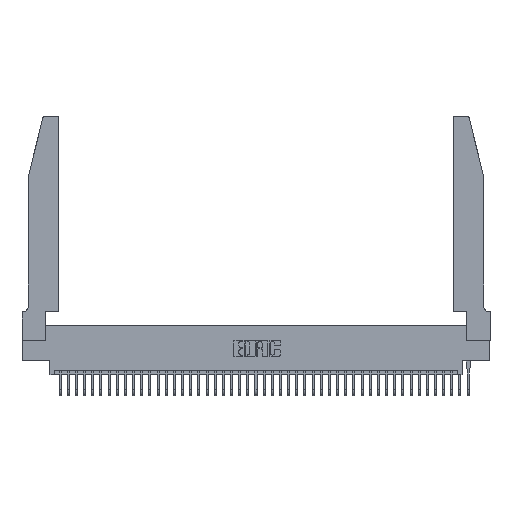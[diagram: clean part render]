
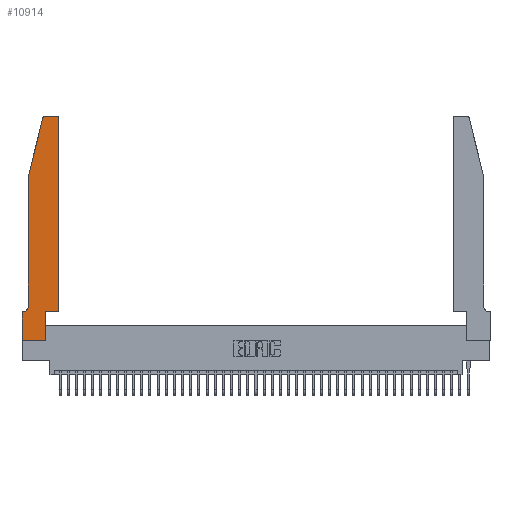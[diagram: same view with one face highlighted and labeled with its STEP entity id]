
A CAD part, top view. The second image highlights one B-rep face of the part: STEP entity #10914.
In plain terms, the highlighted planar face has unit normal (0, 0, 1).
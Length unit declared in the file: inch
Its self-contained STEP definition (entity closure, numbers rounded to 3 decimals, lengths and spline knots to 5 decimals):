
#452 = CARTESIAN_POINT ( 'NONE',  ( 0.0055, 0.35, 0.37 ) ) ;
#762 = EDGE_CURVE ( 'NONE', #5723, #13962, #36899, .T. ) ;
#776 = VERTEX_POINT ( 'NONE', #13655 ) ;
#2385 = DIRECTION ( 'NONE',  ( 1., 0., 0. ) ) ;
#2672 = CIRCLE ( 'NONE', #35893, 0.03 ) ;
#3003 = ORIENTED_EDGE ( 'NONE', *, *, #762, .T. ) ;
#4934 = EDGE_CURVE ( 'NONE', #37605, #13787, #37112, .T. ) ;
#5388 = ORIENTED_EDGE ( 'NONE', *, *, #30100, .T. ) ;
#5570 = VECTOR ( 'NONE', #32090, 39.37008 ) ;
#5597 = EDGE_CURVE ( 'NONE', #13962, #30476, #32188, .T. ) ;
#5723 = VERTEX_POINT ( 'NONE', #16733 ) ;
#6811 = ORIENTED_EDGE ( 'NONE', *, *, #8704, .T. ) ;
#6964 = VECTOR ( 'NONE', #10161, 39.37008 ) ;
#7181 = AXIS2_PLACEMENT_3D ( 'NONE', #8800, #21561, #2385 ) ;
#7262 = ORIENTED_EDGE ( 'NONE', *, *, #23439, .T. ) ;
#7342 = VECTOR ( 'NONE', #17781, 39.37008 ) ;
#8704 = EDGE_CURVE ( 'NONE', #13787, #10696, #13478, .T. ) ;
#8800 = CARTESIAN_POINT ( 'NONE',  ( 0., 0.35, 0.37 ) ) ;
#9521 = CARTESIAN_POINT ( 'NONE',  ( 0.284, 2.72, 0.37 ) ) ;
#9686 = VECTOR ( 'NONE', #13775, 39.37008 ) ;
#10075 = CARTESIAN_POINT ( 'NONE',  ( 0.284, 2.75, 0.37 ) ) ;
#10147 = CARTESIAN_POINT ( 'NONE',  ( 0.4505, 0.35, 0.37 ) ) ;
#10161 = DIRECTION ( 'NONE',  ( -1., 0., 0. ) ) ;
#10356 = VECTOR ( 'NONE', #30789, 39.37008 ) ;
#10497 = ORIENTED_EDGE ( 'NONE', *, *, #40943, .T. ) ;
#10669 = LINE ( 'NONE', #13637, #9686 ) ;
#10696 = VERTEX_POINT ( 'NONE', #14131 ) ;
#10909 = EDGE_CURVE ( 'NONE', #776, #25133, #19751, .T. ) ;
#10914 = ADVANCED_FACE ( 'NONE', ( #36312 ), #12021, .T. ) ;
#11039 = ORIENTED_EDGE ( 'NONE', *, *, #29317, .T. ) ;
#11155 = VERTEX_POINT ( 'NONE', #25811 ) ;
#11218 = ORIENTED_EDGE ( 'NONE', *, *, #27161, .T. ) ;
#11342 = LINE ( 'NONE', #40003, #10356 ) ;
#11932 = VERTEX_POINT ( 'NONE', #19848 ) ;
#12021 = PLANE ( 'NONE',  #7181 ) ;
#12068 = DIRECTION ( 'NONE',  ( 0., 0., 1. ) ) ;
#12710 = DIRECTION ( 'NONE',  ( 1., 0., 0. ) ) ;
#12932 = VECTOR ( 'NONE', #19146, 39.37008 ) ;
#13346 = CARTESIAN_POINT ( 'NONE',  ( 0.0755, 0.35, 0.37 ) ) ;
#13478 = LINE ( 'NONE', #14760, #29183 ) ;
#13637 = CARTESIAN_POINT ( 'NONE',  ( 0.2865, 0.35, 0.37 ) ) ;
#13655 = CARTESIAN_POINT ( 'NONE',  ( 0.0755, 0.42, 0.37 ) ) ;
#13775 = DIRECTION ( 'NONE',  ( 0., 1., 0. ) ) ;
#13787 = VERTEX_POINT ( 'NONE', #37447 ) ;
#13962 = VERTEX_POINT ( 'NONE', #16564 ) ;
#14131 = CARTESIAN_POINT ( 'NONE',  ( 0.4505, 2.72, 0.37 ) ) ;
#14760 = CARTESIAN_POINT ( 'NONE',  ( 0.4505, 0.35, 0.37 ) ) ;
#15422 = DIRECTION ( 'NONE',  ( -1., 0., 0. ) ) ;
#16564 = CARTESIAN_POINT ( 'NONE',  ( 0., 0., 0.37 ) ) ;
#16733 = CARTESIAN_POINT ( 'NONE',  ( 0., 0.35, 0.37 ) ) ;
#17781 = DIRECTION ( 'NONE',  ( -0.239, -0.971, 0. ) ) ;
#18431 = DIRECTION ( 'NONE',  ( 0., 0., -1. ) ) ;
#18653 = EDGE_CURVE ( 'NONE', #26326, #11155, #26989, .T. ) ;
#19146 = DIRECTION ( 'NONE',  ( 0., -1., 0. ) ) ;
#19384 = DIRECTION ( 'NONE',  ( 1., 0., 0. ) ) ;
#19490 = VECTOR ( 'NONE', #15422, 39.37008 ) ;
#19751 = CIRCLE ( 'NONE', #39539, 0.07 ) ;
#19848 = CARTESIAN_POINT ( 'NONE',  ( 0.0755, 2., 0.37 ) ) ;
#21561 = DIRECTION ( 'NONE',  ( 0., 0., 1. ) ) ;
#22442 = LINE ( 'NONE', #27901, #19490 ) ;
#22860 = ORIENTED_EDGE ( 'NONE', *, *, #5597, .T. ) ;
#23018 = EDGE_LOOP ( 'NONE', ( #10497, #25179, #11039, #7262, #34843, #11218, #3003, #22860, #30394, #24170, #6811, #5388 ) ) ;
#23439 = EDGE_CURVE ( 'NONE', #11932, #776, #11342, .T. ) ;
#23904 = CARTESIAN_POINT ( 'NONE',  ( 0.4205, 2.75, 0.37 ) ) ;
#23949 = CARTESIAN_POINT ( 'NONE',  ( 0.0755, 2., 0.37 ) ) ;
#24170 = ORIENTED_EDGE ( 'NONE', *, *, #4934, .T. ) ;
#24412 = AXIS2_PLACEMENT_3D ( 'NONE', #9521, #31472, #12710 ) ;
#25133 = VERTEX_POINT ( 'NONE', #452 ) ;
#25179 = ORIENTED_EDGE ( 'NONE', *, *, #18653, .T. ) ;
#25811 = CARTESIAN_POINT ( 'NONE',  ( 0.25487, 2.72718, 0.37 ) ) ;
#26326 = VERTEX_POINT ( 'NONE', #10075 ) ;
#26375 = CARTESIAN_POINT ( 'NONE',  ( 0.2865, 0., 0.37 ) ) ;
#26989 = CIRCLE ( 'NONE', #24412, 0.03 ) ;
#27161 = EDGE_CURVE ( 'NONE', #25133, #5723, #32109, .T. ) ;
#27901 = CARTESIAN_POINT ( 'NONE',  ( 0.2605, 2.75, 0.37 ) ) ;
#28403 = CARTESIAN_POINT ( 'NONE',  ( 0., 0., 0.37 ) ) ;
#28669 = CARTESIAN_POINT ( 'NONE',  ( 0., 0., 0.37 ) ) ;
#29183 = VECTOR ( 'NONE', #30342, 39.37008 ) ;
#29317 = EDGE_CURVE ( 'NONE', #11155, #11932, #32477, .T. ) ;
#30100 = EDGE_CURVE ( 'NONE', #10696, #33135, #2672, .T. ) ;
#30342 = DIRECTION ( 'NONE',  ( 0., 1., 0. ) ) ;
#30394 = ORIENTED_EDGE ( 'NONE', *, *, #38773, .T. ) ;
#30476 = VERTEX_POINT ( 'NONE', #26375 ) ;
#30610 = CARTESIAN_POINT ( 'NONE',  ( 0.2865, 0.35, 0.37 ) ) ;
#30789 = DIRECTION ( 'NONE',  ( 0., -1., 0. ) ) ;
#30844 = CARTESIAN_POINT ( 'NONE',  ( 0.4205, 2.72, 0.37 ) ) ;
#31472 = DIRECTION ( 'NONE',  ( 0., 0., 1. ) ) ;
#32090 = DIRECTION ( 'NONE',  ( 1., 0., 0. ) ) ;
#32109 = LINE ( 'NONE', #13346, #6964 ) ;
#32188 = LINE ( 'NONE', #28669, #38474 ) ;
#32477 = LINE ( 'NONE', #23949, #7342 ) ;
#33135 = VERTEX_POINT ( 'NONE', #23904 ) ;
#34002 = DIRECTION ( 'NONE',  ( 1., 0., 0. ) ) ;
#34843 = ORIENTED_EDGE ( 'NONE', *, *, #10909, .T. ) ;
#35893 = AXIS2_PLACEMENT_3D ( 'NONE', #30844, #12068, #34002 ) ;
#36312 = FACE_OUTER_BOUND ( 'NONE', #23018, .T. ) ;
#36899 = LINE ( 'NONE', #28403, #12932 ) ;
#37075 = CARTESIAN_POINT ( 'NONE',  ( 0.0055, 0.42, 0.37 ) ) ;
#37112 = LINE ( 'NONE', #10147, #5570 ) ;
#37447 = CARTESIAN_POINT ( 'NONE',  ( 0.4505, 0.35, 0.37 ) ) ;
#37605 = VERTEX_POINT ( 'NONE', #30610 ) ;
#38474 = VECTOR ( 'NONE', #19384, 39.37008 ) ;
#38773 = EDGE_CURVE ( 'NONE', #30476, #37605, #10669, .T. ) ;
#39539 = AXIS2_PLACEMENT_3D ( 'NONE', #37075, #18431, #40166 ) ;
#40003 = CARTESIAN_POINT ( 'NONE',  ( 0.0755, 2., 0.37 ) ) ;
#40166 = DIRECTION ( 'NONE',  ( -1., 0., 0. ) ) ;
#40943 = EDGE_CURVE ( 'NONE', #33135, #26326, #22442, .T. ) ;
